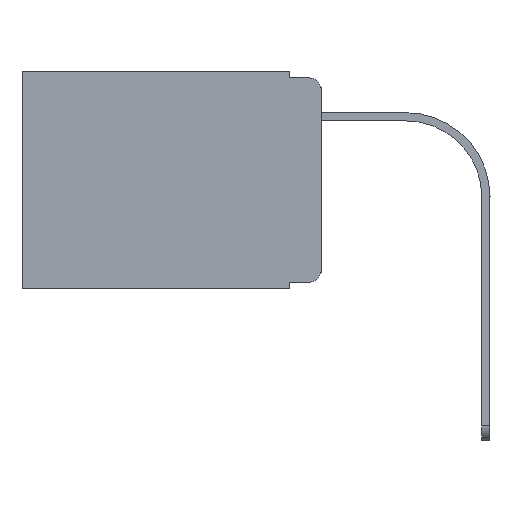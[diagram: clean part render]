
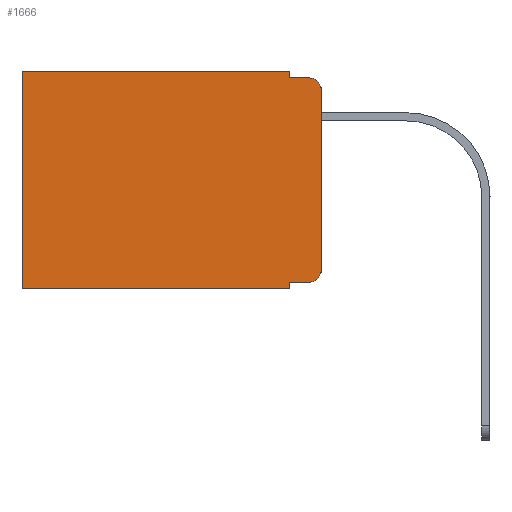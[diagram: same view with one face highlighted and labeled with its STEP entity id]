
A CAD part, left-side view. The second image highlights one B-rep face of the part: STEP entity #1666.
In plain terms, the highlighted planar face has unit normal (-1, 0, 0).
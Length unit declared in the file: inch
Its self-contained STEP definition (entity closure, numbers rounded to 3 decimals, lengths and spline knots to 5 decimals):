
#35 = VECTOR ( 'NONE', #15282, 39.37008 ) ;
#321 = CARTESIAN_POINT ( 'NONE',  ( 0.298, 0.02, -0.313 ) ) ;
#373 = EDGE_CURVE ( 'NONE', #551, #13006, #6976, .T. ) ;
#551 = VERTEX_POINT ( 'NONE', #9718 ) ;
#1025 = EDGE_CURVE ( 'NONE', #14251, #12014, #12403, .T. ) ;
#1139 = CARTESIAN_POINT ( 'NONE',  ( 0.298, 0.051, -0.01 ) ) ;
#1263 = DIRECTION ( 'NONE',  ( 0., 0., -1. ) ) ;
#1531 = VECTOR ( 'NONE', #10824, 39.37008 ) ;
#1649 = CARTESIAN_POINT ( 'NONE',  ( 0.298, 0.473, -0.343 ) ) ;
#1666 = ADVANCED_FACE ( 'NONE', ( #2482 ), #11757, .F. ) ;
#1677 = LINE ( 'NONE', #4047, #8893 ) ;
#1803 = ORIENTED_EDGE ( 'NONE', *, *, #6508, .T. ) ;
#1894 = VECTOR ( 'NONE', #5472, 39.37008 ) ;
#2003 = CARTESIAN_POINT ( 'NONE',  ( 0.298, 0., -0.343 ) ) ;
#2125 = EDGE_CURVE ( 'NONE', #10635, #9283, #1677, .T. ) ;
#2194 = ORIENTED_EDGE ( 'NONE', *, *, #7907, .F. ) ;
#2303 = ORIENTED_EDGE ( 'NONE', *, *, #1025, .F. ) ;
#2482 = FACE_OUTER_BOUND ( 'NONE', #3157, .T. ) ;
#2502 = CARTESIAN_POINT ( 'NONE',  ( 0.298, 0., 0. ) ) ;
#2527 = EDGE_CURVE ( 'NONE', #14450, #14613, #12359, .T. ) ;
#2582 = CARTESIAN_POINT ( 'NONE',  ( 0.298, 0.051, -0.01 ) ) ;
#2716 = CARTESIAN_POINT ( 'NONE',  ( 0.298, 0.051, -0.333 ) ) ;
#2932 = ORIENTED_EDGE ( 'NONE', *, *, #12817, .T. ) ;
#3157 = EDGE_LOOP ( 'NONE', ( #2194, #14041, #6595, #14227, #1803, #7095, #9580, #2303, #2932, #14779 ) ) ;
#3306 = EDGE_CURVE ( 'NONE', #9283, #14613, #7203, .T. ) ;
#3473 = DIRECTION ( 'NONE',  ( 0., 0., -1. ) ) ;
#3547 = DIRECTION ( 'NONE',  ( -1., 0., 0. ) ) ;
#3595 = AXIS2_PLACEMENT_3D ( 'NONE', #321, #3547, #1263 ) ;
#3722 = LINE ( 'NONE', #2502, #11715 ) ;
#3732 = DIRECTION ( 'NONE',  ( 0., -1., 0. ) ) ;
#3885 = EDGE_CURVE ( 'NONE', #12014, #13006, #7925, .T. ) ;
#3895 = DIRECTION ( 'NONE',  ( 0., 0., -1. ) ) ;
#4047 = CARTESIAN_POINT ( 'NONE',  ( 0.298, 0.051, 0. ) ) ;
#4338 = CIRCLE ( 'NONE', #3595, 0.02 ) ;
#4386 = DIRECTION ( 'NONE',  ( 0., 1., 0. ) ) ;
#4766 = CARTESIAN_POINT ( 'NONE',  ( 0.298, 0., 0. ) ) ;
#5472 = DIRECTION ( 'NONE',  ( 0., 0., -1. ) ) ;
#5690 = AXIS2_PLACEMENT_3D ( 'NONE', #9286, #10438, #11437 ) ;
#5944 = VERTEX_POINT ( 'NONE', #12597 ) ;
#6047 = VECTOR ( 'NONE', #4386, 39.37008 ) ;
#6508 = EDGE_CURVE ( 'NONE', #10635, #551, #3722, .T. ) ;
#6595 = ORIENTED_EDGE ( 'NONE', *, *, #3306, .F. ) ;
#6731 = CARTESIAN_POINT ( 'NONE',  ( 0.298, 0.051, 0. ) ) ;
#6929 = CARTESIAN_POINT ( 'NONE',  ( 0.298, 0., 0. ) ) ;
#6976 = LINE ( 'NONE', #7977, #35 ) ;
#7095 = ORIENTED_EDGE ( 'NONE', *, *, #373, .T. ) ;
#7196 = DIRECTION ( 'NONE',  ( 0., 1., 0. ) ) ;
#7203 = LINE ( 'NONE', #1139, #10234 ) ;
#7600 = EDGE_CURVE ( 'NONE', #8321, #5944, #4338, .T. ) ;
#7742 = DIRECTION ( 'NONE',  ( 0., 0., -1. ) ) ;
#7907 = EDGE_CURVE ( 'NONE', #14450, #5944, #9193, .T. ) ;
#7925 = LINE ( 'NONE', #2003, #6047 ) ;
#7977 = CARTESIAN_POINT ( 'NONE',  ( 0.298, 0.473, 0. ) ) ;
#8321 = VERTEX_POINT ( 'NONE', #14827 ) ;
#8893 = VECTOR ( 'NONE', #7742, 39.37008 ) ;
#8907 = CARTESIAN_POINT ( 'NONE',  ( 0.298, 0.02, -0.01 ) ) ;
#9122 = AXIS2_PLACEMENT_3D ( 'NONE', #4766, #10445, #3473 ) ;
#9193 = LINE ( 'NONE', #6929, #1894 ) ;
#9283 = VERTEX_POINT ( 'NONE', #2582 ) ;
#9286 = CARTESIAN_POINT ( 'NONE',  ( 0.298, 0.02, -0.03 ) ) ;
#9580 = ORIENTED_EDGE ( 'NONE', *, *, #3885, .F. ) ;
#9595 = LINE ( 'NONE', #13372, #1531 ) ;
#9718 = CARTESIAN_POINT ( 'NONE',  ( 0.298, 0.473, 0. ) ) ;
#10234 = VECTOR ( 'NONE', #3732, 39.37008 ) ;
#10386 = CARTESIAN_POINT ( 'NONE',  ( 0.298, 0.051, -0.343 ) ) ;
#10438 = DIRECTION ( 'NONE',  ( -1., 0., 0. ) ) ;
#10445 = DIRECTION ( 'NONE',  ( 1., 0., 0. ) ) ;
#10635 = VERTEX_POINT ( 'NONE', #6731 ) ;
#10824 = DIRECTION ( 'NONE',  ( 0., -1., 0. ) ) ;
#11437 = DIRECTION ( 'NONE',  ( 0., 0., -1. ) ) ;
#11715 = VECTOR ( 'NONE', #7196, 39.37008 ) ;
#11757 = PLANE ( 'NONE',  #9122 ) ;
#12014 = VERTEX_POINT ( 'NONE', #10386 ) ;
#12076 = CARTESIAN_POINT ( 'NONE',  ( 0.298, 0., -0.03 ) ) ;
#12086 = CARTESIAN_POINT ( 'NONE',  ( 0.298, 0.051, 0. ) ) ;
#12359 = CIRCLE ( 'NONE', #5690, 0.02 ) ;
#12403 = LINE ( 'NONE', #12086, #14826 ) ;
#12597 = CARTESIAN_POINT ( 'NONE',  ( 0.298, 0., -0.313 ) ) ;
#12817 = EDGE_CURVE ( 'NONE', #14251, #8321, #9595, .T. ) ;
#13006 = VERTEX_POINT ( 'NONE', #1649 ) ;
#13372 = CARTESIAN_POINT ( 'NONE',  ( 0.298, 0.051, -0.333 ) ) ;
#14041 = ORIENTED_EDGE ( 'NONE', *, *, #2527, .T. ) ;
#14227 = ORIENTED_EDGE ( 'NONE', *, *, #2125, .F. ) ;
#14251 = VERTEX_POINT ( 'NONE', #2716 ) ;
#14450 = VERTEX_POINT ( 'NONE', #12076 ) ;
#14613 = VERTEX_POINT ( 'NONE', #8907 ) ;
#14779 = ORIENTED_EDGE ( 'NONE', *, *, #7600, .T. ) ;
#14826 = VECTOR ( 'NONE', #3895, 39.37008 ) ;
#14827 = CARTESIAN_POINT ( 'NONE',  ( 0.298, 0.02, -0.333 ) ) ;
#15282 = DIRECTION ( 'NONE',  ( 0., 0., -1. ) ) ;
